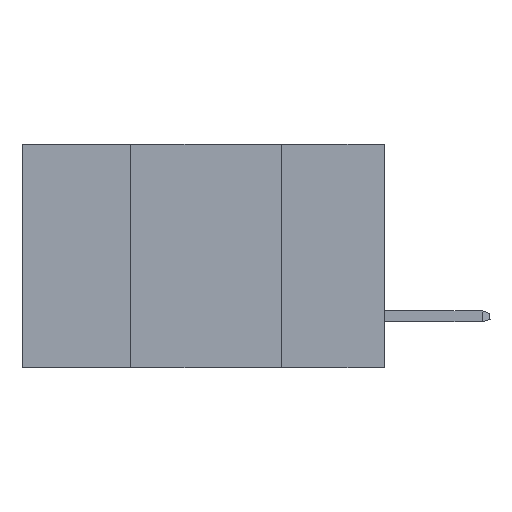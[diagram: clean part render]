
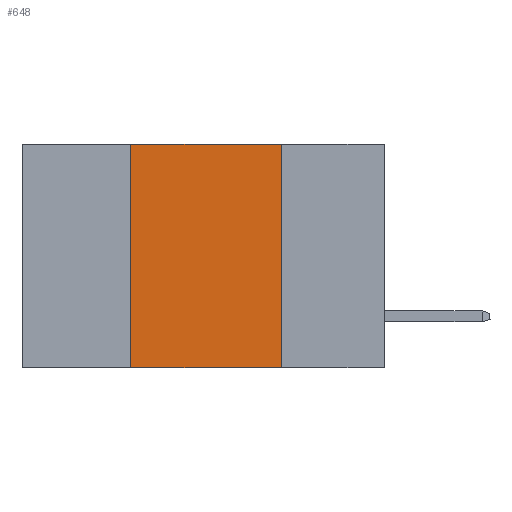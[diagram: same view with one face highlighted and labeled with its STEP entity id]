
A CAD part, left-side view. The second image highlights one B-rep face of the part: STEP entity #648.
In plain terms, the highlighted planar face has unit normal (-1, 0, 0).
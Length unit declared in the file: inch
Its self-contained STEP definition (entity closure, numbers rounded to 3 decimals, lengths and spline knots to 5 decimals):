
#51 = LINE ( 'NONE', #7230, #885 ) ;
#648 = ADVANCED_FACE ( 'NONE', ( #7964 ), #5638, .F. ) ;
#778 = ORIENTED_EDGE ( 'NONE', *, *, #9993, .F. ) ;
#867 = DIRECTION ( 'NONE',  ( 0., -1., 0. ) ) ;
#885 = VECTOR ( 'NONE', #1795, 39.37008 ) ;
#1795 = DIRECTION ( 'NONE',  ( 0., -1., 0. ) ) ;
#2216 = VERTEX_POINT ( 'NONE', #8757 ) ;
#2455 = LINE ( 'NONE', #7173, #2889 ) ;
#2507 = EDGE_CURVE ( 'NONE', #4666, #2216, #9774, .T. ) ;
#2817 = VERTEX_POINT ( 'NONE', #5856 ) ;
#2889 = VECTOR ( 'NONE', #5567, 39.37008 ) ;
#2924 = VECTOR ( 'NONE', #867, 39.37008 ) ;
#2958 = CARTESIAN_POINT ( 'NONE',  ( 0., 0.42, -0.37 ) ) ;
#3052 = VECTOR ( 'NONE', #9212, 39.37008 ) ;
#3214 = AXIS2_PLACEMENT_3D ( 'NONE', #8403, #9202, #3730 ) ;
#3651 = EDGE_CURVE ( 'NONE', #4666, #7356, #2455, .T. ) ;
#3730 = DIRECTION ( 'NONE',  ( 0., 0., -1. ) ) ;
#3981 = ORIENTED_EDGE ( 'NONE', *, *, #7854, .F. ) ;
#4338 = ORIENTED_EDGE ( 'NONE', *, *, #2507, .T. ) ;
#4666 = VERTEX_POINT ( 'NONE', #2958 ) ;
#4706 = CARTESIAN_POINT ( 'NONE',  ( 0., 0.17, 0. ) ) ;
#5567 = DIRECTION ( 'NONE',  ( 0., 0., 1. ) ) ;
#5638 = PLANE ( 'NONE',  #3214 ) ;
#5856 = CARTESIAN_POINT ( 'NONE',  ( 0., 0.17, 0. ) ) ;
#7173 = CARTESIAN_POINT ( 'NONE',  ( 0., 0.42, 0. ) ) ;
#7230 = CARTESIAN_POINT ( 'NONE',  ( 0., 0.6, 0. ) ) ;
#7356 = VERTEX_POINT ( 'NONE', #7949 ) ;
#7854 = EDGE_CURVE ( 'NONE', #2817, #2216, #11756, .T. ) ;
#7949 = CARTESIAN_POINT ( 'NONE',  ( 0., 0.42, 0. ) ) ;
#7964 = FACE_OUTER_BOUND ( 'NONE', #8011, .T. ) ;
#8011 = EDGE_LOOP ( 'NONE', ( #3981, #778, #8044, #4338 ) ) ;
#8044 = ORIENTED_EDGE ( 'NONE', *, *, #3651, .F. ) ;
#8403 = CARTESIAN_POINT ( 'NONE',  ( 0., 0.6, 0. ) ) ;
#8757 = CARTESIAN_POINT ( 'NONE',  ( 0., 0.17, -0.37 ) ) ;
#9148 = CARTESIAN_POINT ( 'NONE',  ( 0., 0.6, -0.37 ) ) ;
#9202 = DIRECTION ( 'NONE',  ( 1., 0., 0. ) ) ;
#9212 = DIRECTION ( 'NONE',  ( 0., 0., -1. ) ) ;
#9774 = LINE ( 'NONE', #9148, #2924 ) ;
#9993 = EDGE_CURVE ( 'NONE', #7356, #2817, #51, .T. ) ;
#11756 = LINE ( 'NONE', #4706, #3052 ) ;
